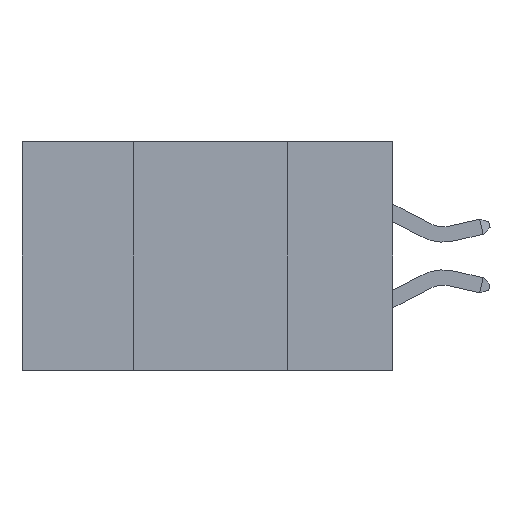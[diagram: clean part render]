
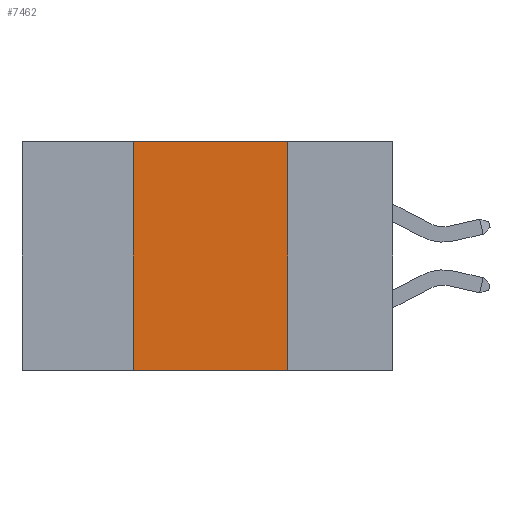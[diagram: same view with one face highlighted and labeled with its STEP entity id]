
A CAD part, left-side view. The second image highlights one B-rep face of the part: STEP entity #7462.
In plain terms, the highlighted planar face has unit normal (-1, 0, 0).
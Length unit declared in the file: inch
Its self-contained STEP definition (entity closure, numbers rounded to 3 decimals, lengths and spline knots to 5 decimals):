
#57 = ORIENTED_EDGE ( 'NONE', *, *, #9013, .F. ) ;
#476 = CARTESIAN_POINT ( 'NONE',  ( 0., 0.42, -0.37 ) ) ;
#842 = CARTESIAN_POINT ( 'NONE',  ( 0., 0.6, -0.37 ) ) ;
#954 = VERTEX_POINT ( 'NONE', #11715 ) ;
#2166 = DIRECTION ( 'NONE',  ( 0., -1., 0. ) ) ;
#2468 = VERTEX_POINT ( 'NONE', #476 ) ;
#2849 = LINE ( 'NONE', #4543, #13309 ) ;
#2914 = CARTESIAN_POINT ( 'NONE',  ( 0., 0.17, 0. ) ) ;
#4543 = CARTESIAN_POINT ( 'NONE',  ( 0., 0.6, 0. ) ) ;
#5192 = VERTEX_POINT ( 'NONE', #8475 ) ;
#5296 = AXIS2_PLACEMENT_3D ( 'NONE', #7844, #16898, #9148 ) ;
#6490 = FACE_OUTER_BOUND ( 'NONE', #15813, .T. ) ;
#6645 = LINE ( 'NONE', #2914, #12749 ) ;
#7247 = EDGE_CURVE ( 'NONE', #2468, #5192, #10178, .T. ) ;
#7462 = ADVANCED_FACE ( 'NONE', ( #6490 ), #15587, .F. ) ;
#7844 = CARTESIAN_POINT ( 'NONE',  ( 0., 0.6, 0. ) ) ;
#8139 = EDGE_CURVE ( 'NONE', #2468, #954, #9328, .T. ) ;
#8475 = CARTESIAN_POINT ( 'NONE',  ( 0., 0.17, -0.37 ) ) ;
#9013 = EDGE_CURVE ( 'NONE', #10733, #5192, #6645, .T. ) ;
#9148 = DIRECTION ( 'NONE',  ( 0., 0., -1. ) ) ;
#9328 = LINE ( 'NONE', #14204, #16216 ) ;
#10178 = LINE ( 'NONE', #842, #16655 ) ;
#10217 = ORIENTED_EDGE ( 'NONE', *, *, #14423, .F. ) ;
#10733 = VERTEX_POINT ( 'NONE', #15234 ) ;
#10736 = DIRECTION ( 'NONE',  ( 0., 0., -1. ) ) ;
#11658 = DIRECTION ( 'NONE',  ( 0., 0., 1. ) ) ;
#11715 = CARTESIAN_POINT ( 'NONE',  ( 0., 0.42, 0. ) ) ;
#12383 = ORIENTED_EDGE ( 'NONE', *, *, #7247, .T. ) ;
#12749 = VECTOR ( 'NONE', #10736, 39.37008 ) ;
#13309 = VECTOR ( 'NONE', #14966, 39.37008 ) ;
#14204 = CARTESIAN_POINT ( 'NONE',  ( 0., 0.42, 0. ) ) ;
#14423 = EDGE_CURVE ( 'NONE', #954, #10733, #2849, .T. ) ;
#14966 = DIRECTION ( 'NONE',  ( 0., -1., 0. ) ) ;
#15234 = CARTESIAN_POINT ( 'NONE',  ( 0., 0.17, 0. ) ) ;
#15587 = PLANE ( 'NONE',  #5296 ) ;
#15813 = EDGE_LOOP ( 'NONE', ( #57, #10217, #16476, #12383 ) ) ;
#16216 = VECTOR ( 'NONE', #11658, 39.37008 ) ;
#16476 = ORIENTED_EDGE ( 'NONE', *, *, #8139, .F. ) ;
#16655 = VECTOR ( 'NONE', #2166, 39.37008 ) ;
#16898 = DIRECTION ( 'NONE',  ( 1., 0., 0. ) ) ;
